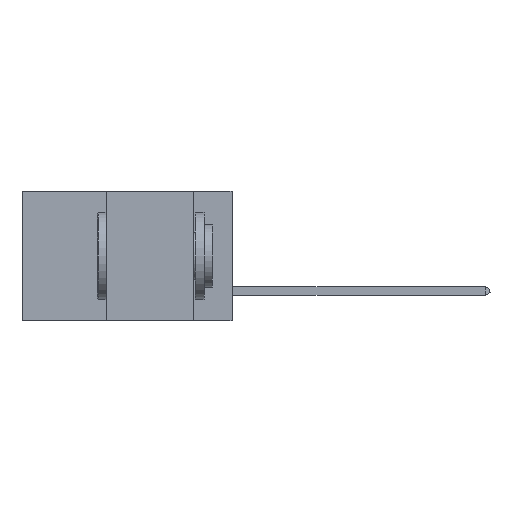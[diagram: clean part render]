
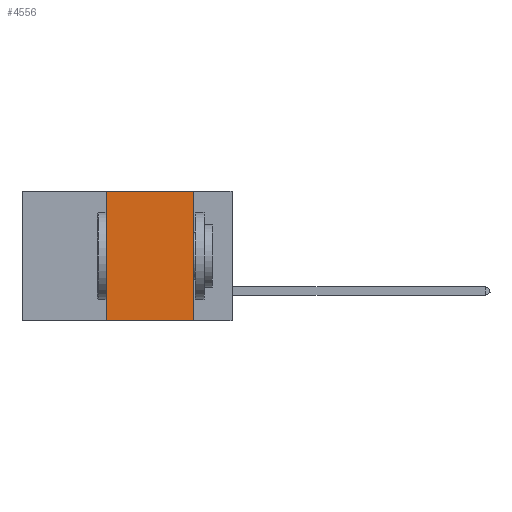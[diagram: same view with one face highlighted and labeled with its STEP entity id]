
A CAD part, left-side view. The second image highlights one B-rep face of the part: STEP entity #4556.
In plain terms, the highlighted planar face has unit normal (-1, 0, 0).
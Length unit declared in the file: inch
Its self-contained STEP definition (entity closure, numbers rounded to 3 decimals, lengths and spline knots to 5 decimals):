
#640 = ORIENTED_EDGE ( 'NONE', *, *, #25949, .F. ) ;
#890 = CARTESIAN_POINT ( 'NONE',  ( 0., 0.11, -0.37 ) ) ;
#3381 = LINE ( 'NONE', #20232, #19552 ) ;
#3573 = VECTOR ( 'NONE', #26091, 39.37008 ) ;
#3730 = LINE ( 'NONE', #17333, #39508 ) ;
#4556 = ADVANCED_FACE ( 'NONE', ( #46709 ), #26561, .F. ) ;
#4713 = DIRECTION ( 'NONE',  ( 0., 0., -1. ) ) ;
#8844 = LINE ( 'NONE', #9637, #47063 ) ;
#9637 = CARTESIAN_POINT ( 'NONE',  ( 0., 0.6, -0.37 ) ) ;
#11389 = EDGE_CURVE ( 'NONE', #36390, #35659, #3730, .T. ) ;
#11769 = DIRECTION ( 'NONE',  ( 1., 0., 0. ) ) ;
#12145 = LINE ( 'NONE', #40582, #3573 ) ;
#13954 = ORIENTED_EDGE ( 'NONE', *, *, #11389, .F. ) ;
#16637 = CARTESIAN_POINT ( 'NONE',  ( 0., 0.36, -0.37 ) ) ;
#17333 = CARTESIAN_POINT ( 'NONE',  ( 0., 0.36, 0. ) ) ;
#19552 = VECTOR ( 'NONE', #45865, 39.37008 ) ;
#20047 = ORIENTED_EDGE ( 'NONE', *, *, #24127, .F. ) ;
#20232 = CARTESIAN_POINT ( 'NONE',  ( 0., 0.11, 0. ) ) ;
#20436 = ORIENTED_EDGE ( 'NONE', *, *, #43956, .T. ) ;
#20818 = EDGE_LOOP ( 'NONE', ( #640, #20047, #13954, #20436 ) ) ;
#20915 = DIRECTION ( 'NONE',  ( 0., 0., 1. ) ) ;
#22970 = CARTESIAN_POINT ( 'NONE',  ( 0., 0.36, 0. ) ) ;
#23197 = CARTESIAN_POINT ( 'NONE',  ( 0., 0.6, 0. ) ) ;
#24127 = EDGE_CURVE ( 'NONE', #35659, #28253, #12145, .T. ) ;
#25949 = EDGE_CURVE ( 'NONE', #28253, #38783, #3381, .T. ) ;
#26091 = DIRECTION ( 'NONE',  ( 0., -1., 0. ) ) ;
#26561 = PLANE ( 'NONE',  #34368 ) ;
#28253 = VERTEX_POINT ( 'NONE', #32276 ) ;
#32276 = CARTESIAN_POINT ( 'NONE',  ( 0., 0.11, 0. ) ) ;
#32304 = DIRECTION ( 'NONE',  ( 0., -1., 0. ) ) ;
#34368 = AXIS2_PLACEMENT_3D ( 'NONE', #23197, #11769, #4713 ) ;
#35659 = VERTEX_POINT ( 'NONE', #22970 ) ;
#36390 = VERTEX_POINT ( 'NONE', #16637 ) ;
#38783 = VERTEX_POINT ( 'NONE', #890 ) ;
#39508 = VECTOR ( 'NONE', #20915, 39.37008 ) ;
#40582 = CARTESIAN_POINT ( 'NONE',  ( 0., 0.6, 0. ) ) ;
#43956 = EDGE_CURVE ( 'NONE', #36390, #38783, #8844, .T. ) ;
#45865 = DIRECTION ( 'NONE',  ( 0., 0., -1. ) ) ;
#46709 = FACE_OUTER_BOUND ( 'NONE', #20818, .T. ) ;
#47063 = VECTOR ( 'NONE', #32304, 39.37008 ) ;
